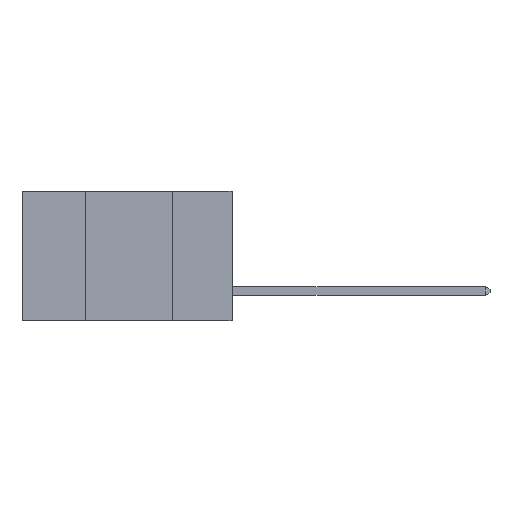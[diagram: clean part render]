
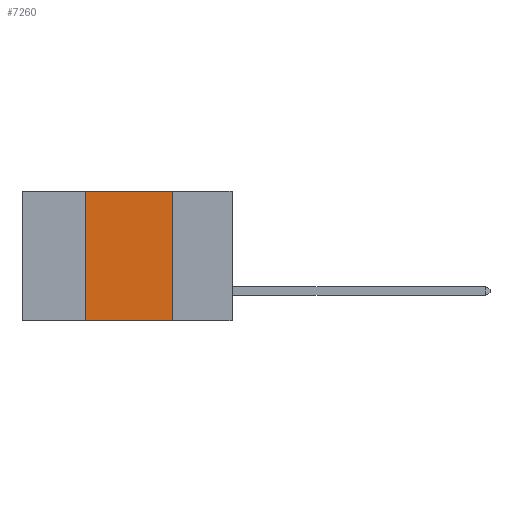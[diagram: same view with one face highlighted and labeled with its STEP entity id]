
A CAD part, left-side view. The second image highlights one B-rep face of the part: STEP entity #7260.
In plain terms, the highlighted planar face has unit normal (-1, 0, 0).
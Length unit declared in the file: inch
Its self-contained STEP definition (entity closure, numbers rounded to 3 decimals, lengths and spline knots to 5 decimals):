
#70 = LINE ( 'NONE', #9047, #2385 ) ;
#479 = CARTESIAN_POINT ( 'NONE',  ( 0., 0.42, 0. ) ) ;
#1098 = EDGE_CURVE ( 'NONE', #6886, #12289, #70, .T. ) ;
#1493 = DIRECTION ( 'NONE',  ( 1., 0., 0. ) ) ;
#1738 = CARTESIAN_POINT ( 'NONE',  ( 0., 0.17, 0. ) ) ;
#2232 = CARTESIAN_POINT ( 'NONE',  ( 0., 0.17, 0. ) ) ;
#2279 = LINE ( 'NONE', #479, #10518 ) ;
#2385 = VECTOR ( 'NONE', #9587, 39.37008 ) ;
#3012 = FACE_OUTER_BOUND ( 'NONE', #12218, .T. ) ;
#3432 = CARTESIAN_POINT ( 'NONE',  ( 0., 0.6, 0. ) ) ;
#3975 = CARTESIAN_POINT ( 'NONE',  ( 0., 0.42, -0.37 ) ) ;
#4903 = EDGE_CURVE ( 'NONE', #5080, #10620, #9033, .T. ) ;
#5080 = VERTEX_POINT ( 'NONE', #8077 ) ;
#5383 = AXIS2_PLACEMENT_3D ( 'NONE', #3432, #1493, #8448 ) ;
#5454 = CARTESIAN_POINT ( 'NONE',  ( 0., 0.17, -0.37 ) ) ;
#6616 = VECTOR ( 'NONE', #11671, 39.37008 ) ;
#6720 = ORIENTED_EDGE ( 'NONE', *, *, #1098, .T. ) ;
#6886 = VERTEX_POINT ( 'NONE', #3975 ) ;
#7260 = ADVANCED_FACE ( 'NONE', ( #3012 ), #7381, .F. ) ;
#7344 = DIRECTION ( 'NONE',  ( 0., 0., 1. ) ) ;
#7381 = PLANE ( 'NONE',  #5383 ) ;
#8077 = CARTESIAN_POINT ( 'NONE',  ( 0., 0.42, 0. ) ) ;
#8129 = LINE ( 'NONE', #1738, #10231 ) ;
#8448 = DIRECTION ( 'NONE',  ( 0., 0., -1. ) ) ;
#8563 = ORIENTED_EDGE ( 'NONE', *, *, #10106, .F. ) ;
#9033 = LINE ( 'NONE', #10800, #6616 ) ;
#9047 = CARTESIAN_POINT ( 'NONE',  ( 0., 0.6, -0.37 ) ) ;
#9054 = EDGE_CURVE ( 'NONE', #10620, #12289, #8129, .T. ) ;
#9392 = DIRECTION ( 'NONE',  ( 0., 0., -1. ) ) ;
#9587 = DIRECTION ( 'NONE',  ( 0., -1., 0. ) ) ;
#10106 = EDGE_CURVE ( 'NONE', #6886, #5080, #2279, .T. ) ;
#10231 = VECTOR ( 'NONE', #9392, 39.37008 ) ;
#10419 = ORIENTED_EDGE ( 'NONE', *, *, #9054, .F. ) ;
#10518 = VECTOR ( 'NONE', #7344, 39.37008 ) ;
#10620 = VERTEX_POINT ( 'NONE', #2232 ) ;
#10703 = ORIENTED_EDGE ( 'NONE', *, *, #4903, .F. ) ;
#10800 = CARTESIAN_POINT ( 'NONE',  ( 0., 0.6, 0. ) ) ;
#11671 = DIRECTION ( 'NONE',  ( 0., -1., 0. ) ) ;
#12218 = EDGE_LOOP ( 'NONE', ( #10419, #10703, #8563, #6720 ) ) ;
#12289 = VERTEX_POINT ( 'NONE', #5454 ) ;
